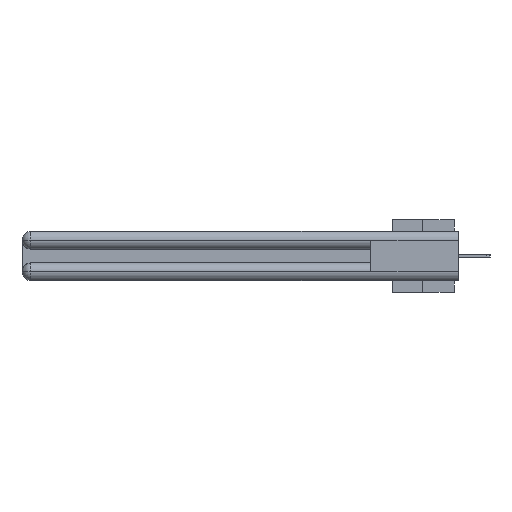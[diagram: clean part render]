
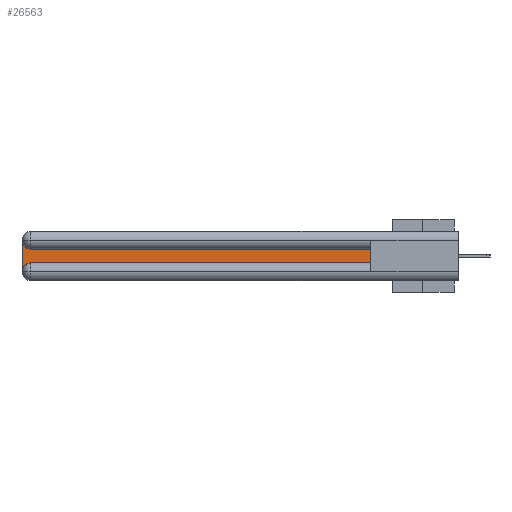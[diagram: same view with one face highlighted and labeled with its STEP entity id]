
A CAD part, left-side view. The second image highlights one B-rep face of the part: STEP entity #26563.
In plain terms, the highlighted planar face has unit normal (-1, 0, 0).
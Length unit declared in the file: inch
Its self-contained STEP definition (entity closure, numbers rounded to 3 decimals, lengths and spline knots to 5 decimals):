
#1612 = VERTEX_POINT ( 'NONE', #31341 ) ;
#2272 = CARTESIAN_POINT ( 'NONE',  ( 0.075, 0.6, -0.1225 ) ) ;
#3397 = PLANE ( 'NONE',  #41325 ) ;
#3983 = LINE ( 'NONE', #2272, #11644 ) ;
#4691 = CIRCLE ( 'NONE', #12731, 0.06 ) ;
#4964 = ORIENTED_EDGE ( 'NONE', *, *, #16847, .T. ) ;
#5162 = DIRECTION ( 'NONE',  ( 1., 0., 0. ) ) ;
#5171 = AXIS2_PLACEMENT_3D ( 'NONE', #24590, #5162, #27818 ) ;
#5585 = DIRECTION ( 'NONE',  ( 0., 1., 0. ) ) ;
#6692 = DIRECTION ( 'NONE',  ( 1., 0., 0. ) ) ;
#8140 = LINE ( 'NONE', #32611, #16725 ) ;
#8372 = ORIENTED_EDGE ( 'NONE', *, *, #9681, .T. ) ;
#9181 = DIRECTION ( 'NONE',  ( 0., -1., 0. ) ) ;
#9638 = VECTOR ( 'NONE', #9181, 39.37008 ) ;
#9681 = EDGE_CURVE ( 'NONE', #19510, #11669, #11450, .T. ) ;
#10128 = DIRECTION ( 'NONE',  ( 0., 0., -1. ) ) ;
#11450 = LINE ( 'NONE', #18148, #27603 ) ;
#11644 = VECTOR ( 'NONE', #5585, 39.37008 ) ;
#11669 = VERTEX_POINT ( 'NONE', #13822 ) ;
#12690 = CARTESIAN_POINT ( 'NONE',  ( 0.075, 2.94, -0.0625 ) ) ;
#12731 = AXIS2_PLACEMENT_3D ( 'NONE', #12690, #35139, #15925 ) ;
#12998 = EDGE_CURVE ( 'NONE', #38271, #28579, #27705, .T. ) ;
#13591 = EDGE_LOOP ( 'NONE', ( #15511, #24877, #4964, #15606, #22341, #8372 ) ) ;
#13822 = CARTESIAN_POINT ( 'NONE',  ( 0.075, 0.6, -0.1225 ) ) ;
#15511 = ORIENTED_EDGE ( 'NONE', *, *, #17423, .T. ) ;
#15606 = ORIENTED_EDGE ( 'NONE', *, *, #12998, .T. ) ;
#15858 = CARTESIAN_POINT ( 'NONE',  ( 0.075, 2.94, -0.2175 ) ) ;
#15925 = DIRECTION ( 'NONE',  ( 0., 0., -1. ) ) ;
#16725 = VECTOR ( 'NONE', #10128, 39.37008 ) ;
#16847 = EDGE_CURVE ( 'NONE', #1612, #38271, #8140, .T. ) ;
#16912 = VERTEX_POINT ( 'NONE', #29825 ) ;
#17423 = EDGE_CURVE ( 'NONE', #11669, #16912, #3983, .T. ) ;
#17501 = EDGE_CURVE ( 'NONE', #28579, #19510, #25772, .T. ) ;
#18148 = CARTESIAN_POINT ( 'NONE',  ( 0.075, 0.6, -0.2175 ) ) ;
#19510 = VERTEX_POINT ( 'NONE', #39530 ) ;
#22175 = CARTESIAN_POINT ( 'NONE',  ( 0.075, 0.6, -0.2175 ) ) ;
#22341 = ORIENTED_EDGE ( 'NONE', *, *, #17501, .T. ) ;
#24590 = CARTESIAN_POINT ( 'NONE',  ( 0.075, 2.94, -0.2775 ) ) ;
#24877 = ORIENTED_EDGE ( 'NONE', *, *, #35324, .T. ) ;
#25772 = LINE ( 'NONE', #22175, #9638 ) ;
#26052 = CARTESIAN_POINT ( 'NONE',  ( 0.075, 3., -0.1225 ) ) ;
#26563 = ADVANCED_FACE ( 'NONE', ( #30126 ), #3397, .F. ) ;
#27603 = VECTOR ( 'NONE', #37301, 39.37008 ) ;
#27705 = CIRCLE ( 'NONE', #5171, 0.06 ) ;
#27818 = DIRECTION ( 'NONE',  ( 0., 0., -1. ) ) ;
#28579 = VERTEX_POINT ( 'NONE', #15858 ) ;
#29285 = DIRECTION ( 'NONE',  ( 0., 0., -1. ) ) ;
#29825 = CARTESIAN_POINT ( 'NONE',  ( 0.075, 2.94, -0.1225 ) ) ;
#30126 = FACE_OUTER_BOUND ( 'NONE', #13591, .T. ) ;
#31341 = CARTESIAN_POINT ( 'NONE',  ( 0.075, 3., -0.0625 ) ) ;
#32611 = CARTESIAN_POINT ( 'NONE',  ( 0.075, 3., -0.2175 ) ) ;
#34087 = CARTESIAN_POINT ( 'NONE',  ( 0.075, 3., -0.2775 ) ) ;
#35139 = DIRECTION ( 'NONE',  ( 1., 0., 0. ) ) ;
#35324 = EDGE_CURVE ( 'NONE', #16912, #1612, #4691, .T. ) ;
#37301 = DIRECTION ( 'NONE',  ( 0., 0., 1. ) ) ;
#38271 = VERTEX_POINT ( 'NONE', #34087 ) ;
#39530 = CARTESIAN_POINT ( 'NONE',  ( 0.075, 0.6, -0.2175 ) ) ;
#41325 = AXIS2_PLACEMENT_3D ( 'NONE', #26052, #6692, #29285 ) ;
